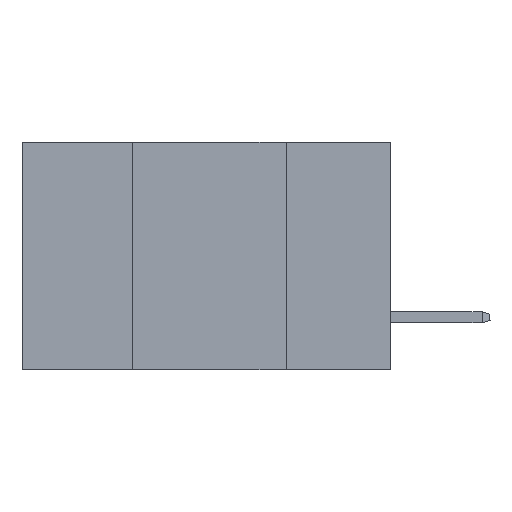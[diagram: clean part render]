
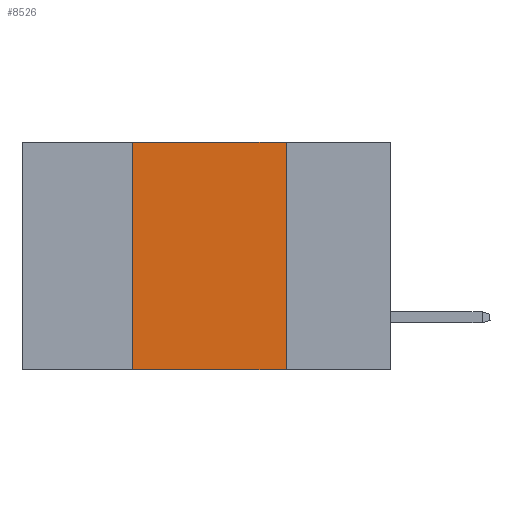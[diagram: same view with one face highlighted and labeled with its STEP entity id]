
A CAD part, left-side view. The second image highlights one B-rep face of the part: STEP entity #8526.
In plain terms, the highlighted planar face has unit normal (-1, 0, 0).
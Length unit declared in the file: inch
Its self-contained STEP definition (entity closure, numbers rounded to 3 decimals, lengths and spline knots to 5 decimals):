
#386 = DIRECTION ( 'NONE',  ( 0., 0., -1. ) ) ;
#394 = DIRECTION ( 'NONE',  ( 0., 0., 1. ) ) ;
#922 = CARTESIAN_POINT ( 'NONE',  ( 0., 0.6, 0. ) ) ;
#1864 = FACE_OUTER_BOUND ( 'NONE', #14030, .T. ) ;
#3483 = LINE ( 'NONE', #13995, #4554 ) ;
#4081 = LINE ( 'NONE', #6755, #14360 ) ;
#4554 = VECTOR ( 'NONE', #386, 39.37008 ) ;
#4691 = PLANE ( 'NONE',  #44515 ) ;
#4909 = LINE ( 'NONE', #37830, #40597 ) ;
#6755 = CARTESIAN_POINT ( 'NONE',  ( 0., 0.42, 0. ) ) ;
#7083 = ORIENTED_EDGE ( 'NONE', *, *, #18441, .F. ) ;
#8526 = ADVANCED_FACE ( 'NONE', ( #1864 ), #4691, .F. ) ;
#9891 = CARTESIAN_POINT ( 'NONE',  ( 0., 0.17, -0.37 ) ) ;
#11017 = VERTEX_POINT ( 'NONE', #28313 ) ;
#11948 = LINE ( 'NONE', #26851, #27100 ) ;
#13995 = CARTESIAN_POINT ( 'NONE',  ( 0., 0.17, 0. ) ) ;
#14030 = EDGE_LOOP ( 'NONE', ( #17110, #7083, #24612, #30181 ) ) ;
#14360 = VECTOR ( 'NONE', #394, 39.37008 ) ;
#17110 = ORIENTED_EDGE ( 'NONE', *, *, #22528, .F. ) ;
#18158 = DIRECTION ( 'NONE',  ( 1., 0., 0. ) ) ;
#18441 = EDGE_CURVE ( 'NONE', #11017, #29777, #11948, .T. ) ;
#18530 = EDGE_CURVE ( 'NONE', #29294, #24757, #4909, .T. ) ;
#20630 = CARTESIAN_POINT ( 'NONE',  ( 0., 0.17, 0. ) ) ;
#22528 = EDGE_CURVE ( 'NONE', #29777, #24757, #3483, .T. ) ;
#23950 = DIRECTION ( 'NONE',  ( 0., -1., 0. ) ) ;
#24612 = ORIENTED_EDGE ( 'NONE', *, *, #33728, .F. ) ;
#24757 = VERTEX_POINT ( 'NONE', #9891 ) ;
#26851 = CARTESIAN_POINT ( 'NONE',  ( 0., 0.6, 0. ) ) ;
#27100 = VECTOR ( 'NONE', #40432, 39.37008 ) ;
#28313 = CARTESIAN_POINT ( 'NONE',  ( 0., 0.42, 0. ) ) ;
#29294 = VERTEX_POINT ( 'NONE', #31718 ) ;
#29777 = VERTEX_POINT ( 'NONE', #20630 ) ;
#30181 = ORIENTED_EDGE ( 'NONE', *, *, #18530, .T. ) ;
#31718 = CARTESIAN_POINT ( 'NONE',  ( 0., 0.42, -0.37 ) ) ;
#33728 = EDGE_CURVE ( 'NONE', #29294, #11017, #4081, .T. ) ;
#35795 = DIRECTION ( 'NONE',  ( 0., 0., -1. ) ) ;
#37830 = CARTESIAN_POINT ( 'NONE',  ( 0., 0.6, -0.37 ) ) ;
#40432 = DIRECTION ( 'NONE',  ( 0., -1., 0. ) ) ;
#40597 = VECTOR ( 'NONE', #23950, 39.37008 ) ;
#44515 = AXIS2_PLACEMENT_3D ( 'NONE', #922, #18158, #35795 ) ;
